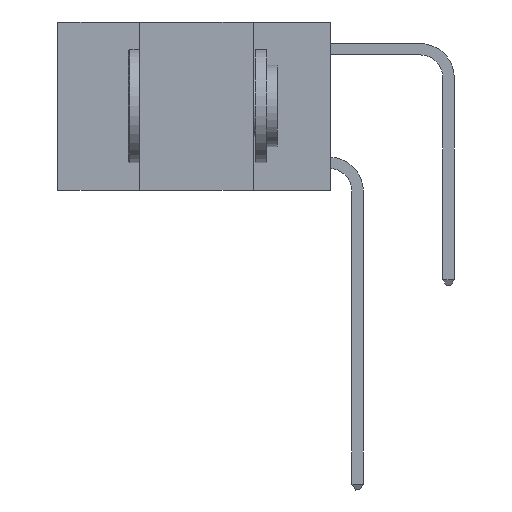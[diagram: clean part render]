
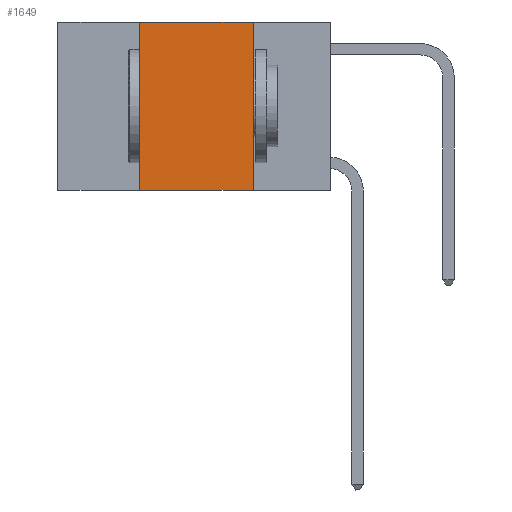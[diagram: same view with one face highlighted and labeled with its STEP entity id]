
A CAD part, left-side view. The second image highlights one B-rep face of the part: STEP entity #1649.
In plain terms, the highlighted planar face has unit normal (-1, 0, 0).
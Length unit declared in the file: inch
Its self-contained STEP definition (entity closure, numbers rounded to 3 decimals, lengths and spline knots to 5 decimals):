
#497 = DIRECTION ( 'NONE',  ( 0., 0., -1. ) ) ;
#869 = PLANE ( 'NONE',  #3296 ) ;
#988 = DIRECTION ( 'NONE',  ( 1., 0., 0. ) ) ;
#1158 = ORIENTED_EDGE ( 'NONE', *, *, #5790, .T. ) ;
#1233 = VERTEX_POINT ( 'NONE', #2884 ) ;
#1292 = ORIENTED_EDGE ( 'NONE', *, *, #9796, .F. ) ;
#1459 = FACE_OUTER_BOUND ( 'NONE', #5365, .T. ) ;
#1526 = ORIENTED_EDGE ( 'NONE', *, *, #6592, .F. ) ;
#1529 = CARTESIAN_POINT ( 'NONE',  ( 0., 0.6, 0. ) ) ;
#1649 = ADVANCED_FACE ( 'NONE', ( #1459 ), #869, .F. ) ;
#2136 = VECTOR ( 'NONE', #5577, 39.37008 ) ;
#2185 = VERTEX_POINT ( 'NONE', #8025 ) ;
#2683 = VECTOR ( 'NONE', #11711, 39.37008 ) ;
#2698 = LINE ( 'NONE', #7515, #7921 ) ;
#2853 = VERTEX_POINT ( 'NONE', #8161 ) ;
#2884 = CARTESIAN_POINT ( 'NONE',  ( 0., 0.17, 0. ) ) ;
#2955 = LINE ( 'NONE', #4302, #2683 ) ;
#3296 = AXIS2_PLACEMENT_3D ( 'NONE', #1529, #988, #497 ) ;
#3517 = CARTESIAN_POINT ( 'NONE',  ( 0., 0.42, 0. ) ) ;
#4302 = CARTESIAN_POINT ( 'NONE',  ( 0., 0.42, 0. ) ) ;
#5365 = EDGE_LOOP ( 'NONE', ( #1526, #1292, #10794, #1158 ) ) ;
#5577 = DIRECTION ( 'NONE',  ( 0., -1., 0. ) ) ;
#5790 = EDGE_CURVE ( 'NONE', #2853, #2185, #9751, .T. ) ;
#5844 = VERTEX_POINT ( 'NONE', #3517 ) ;
#6354 = CARTESIAN_POINT ( 'NONE',  ( 0., 0.6, -0.37 ) ) ;
#6592 = EDGE_CURVE ( 'NONE', #1233, #2185, #2698, .T. ) ;
#6891 = EDGE_CURVE ( 'NONE', #2853, #5844, #2955, .T. ) ;
#6950 = CARTESIAN_POINT ( 'NONE',  ( 0., 0.6, 0. ) ) ;
#7515 = CARTESIAN_POINT ( 'NONE',  ( 0., 0.17, 0. ) ) ;
#7523 = DIRECTION ( 'NONE',  ( 0., -1., 0. ) ) ;
#7921 = VECTOR ( 'NONE', #11079, 39.37008 ) ;
#8025 = CARTESIAN_POINT ( 'NONE',  ( 0., 0.17, -0.37 ) ) ;
#8161 = CARTESIAN_POINT ( 'NONE',  ( 0., 0.42, -0.37 ) ) ;
#9299 = VECTOR ( 'NONE', #7523, 39.37008 ) ;
#9751 = LINE ( 'NONE', #6354, #2136 ) ;
#9796 = EDGE_CURVE ( 'NONE', #5844, #1233, #12103, .T. ) ;
#10794 = ORIENTED_EDGE ( 'NONE', *, *, #6891, .F. ) ;
#11079 = DIRECTION ( 'NONE',  ( 0., 0., -1. ) ) ;
#11711 = DIRECTION ( 'NONE',  ( 0., 0., 1. ) ) ;
#12103 = LINE ( 'NONE', #6950, #9299 ) ;
